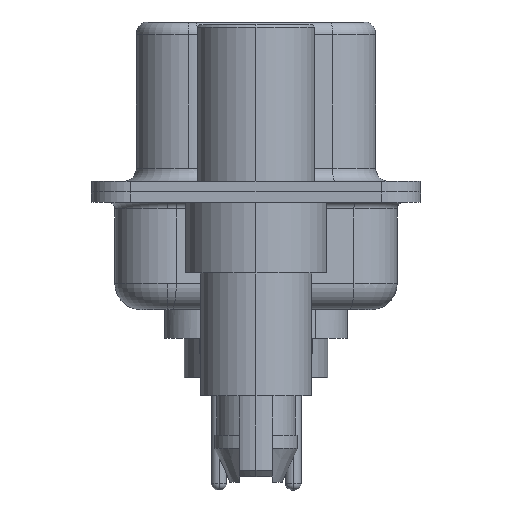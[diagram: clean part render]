
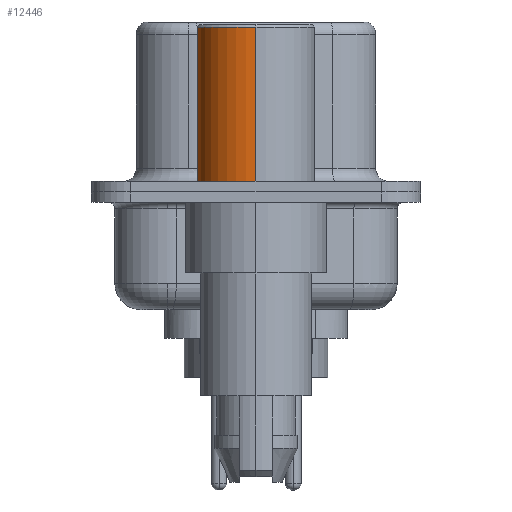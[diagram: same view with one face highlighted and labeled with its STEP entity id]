
A CAD part, left-side view. The second image highlights one B-rep face of the part: STEP entity #12446.
In plain terms, the highlighted cylindrical face has radius 2.25 mm (diameter 4.5 mm), a partial arc.
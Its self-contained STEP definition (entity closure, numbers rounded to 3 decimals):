
#84 = ORIENTED_EDGE ( 'NONE', *, *, #14994, .F. ) ;
#2741 = CARTESIAN_POINT ( 'NONE',  ( 2.25, 0., 0.581 ) ) ;
#2991 = CARTESIAN_POINT ( 'NONE',  ( 2.25, 0., 6.3 ) ) ;
#3329 = LINE ( 'NONE', #4265, #8556 ) ;
#3680 = DIRECTION ( 'NONE',  ( 0., 0., 1. ) ) ;
#3820 = CIRCLE ( 'NONE', #4829, 2.25 ) ;
#4265 = CARTESIAN_POINT ( 'NONE',  ( -2.25, 0., 0.581 ) ) ;
#4718 = VERTEX_POINT ( 'NONE', #2991 ) ;
#4829 = AXIS2_PLACEMENT_3D ( 'NONE', #15387, #5788, #16952 ) ;
#4986 = ORIENTED_EDGE ( 'NONE', *, *, #15563, .T. ) ;
#5249 = AXIS2_PLACEMENT_3D ( 'NONE', #11685, #3680, #19596 ) ;
#5683 = FACE_OUTER_BOUND ( 'NONE', #18584, .T. ) ;
#5788 = DIRECTION ( 'NONE',  ( 0., 0., 1. ) ) ;
#5850 = DIRECTION ( 'NONE',  ( 0., 0., 1. ) ) ;
#6527 = VERTEX_POINT ( 'NONE', #16689 ) ;
#7640 = DIRECTION ( 'NONE',  ( 0., 0., 1. ) ) ;
#7817 = CARTESIAN_POINT ( 'NONE',  ( 2.25, 0., 0.4 ) ) ;
#8319 = ORIENTED_EDGE ( 'NONE', *, *, #15622, .F. ) ;
#8324 = VERTEX_POINT ( 'NONE', #14352 ) ;
#8556 = VECTOR ( 'NONE', #5850, 1000. ) ;
#8915 = CYLINDRICAL_SURFACE ( 'NONE', #5249, 2.25 ) ;
#10219 = VERTEX_POINT ( 'NONE', #7817 ) ;
#10525 = ORIENTED_EDGE ( 'NONE', *, *, #15589, .T. ) ;
#11287 = LINE ( 'NONE', #2741, #15074 ) ;
#11685 = CARTESIAN_POINT ( 'NONE',  ( 0., 0., 0.581 ) ) ;
#11819 = CIRCLE ( 'NONE', #17772, 2.25 ) ;
#12446 = ADVANCED_FACE ( 'NONE', ( #5683 ), #8915, .T. ) ;
#13916 = DIRECTION ( 'NONE',  ( 0., 0., 1. ) ) ;
#14352 = CARTESIAN_POINT ( 'NONE',  ( -2.25, 0., 6.3 ) ) ;
#14994 = EDGE_CURVE ( 'NONE', #4718, #8324, #11819, .T. ) ;
#15074 = VECTOR ( 'NONE', #13916, 1000. ) ;
#15387 = CARTESIAN_POINT ( 'NONE',  ( 0., 0., 0.4 ) ) ;
#15563 = EDGE_CURVE ( 'NONE', #10219, #6527, #3820, .T. ) ;
#15589 = EDGE_CURVE ( 'NONE', #6527, #8324, #3329, .T. ) ;
#15622 = EDGE_CURVE ( 'NONE', #10219, #4718, #11287, .T. ) ;
#16689 = CARTESIAN_POINT ( 'NONE',  ( -2.25, 0., 0.4 ) ) ;
#16952 = DIRECTION ( 'NONE',  ( 1., 0., 0. ) ) ;
#17183 = CARTESIAN_POINT ( 'NONE',  ( 0., 0., 6.3 ) ) ;
#17772 = AXIS2_PLACEMENT_3D ( 'NONE', #17183, #7640, #18753 ) ;
#18584 = EDGE_LOOP ( 'NONE', ( #4986, #10525, #84, #8319 ) ) ;
#18753 = DIRECTION ( 'NONE',  ( 1., 0., 0. ) ) ;
#19596 = DIRECTION ( 'NONE',  ( 1., 0., 0. ) ) ;
